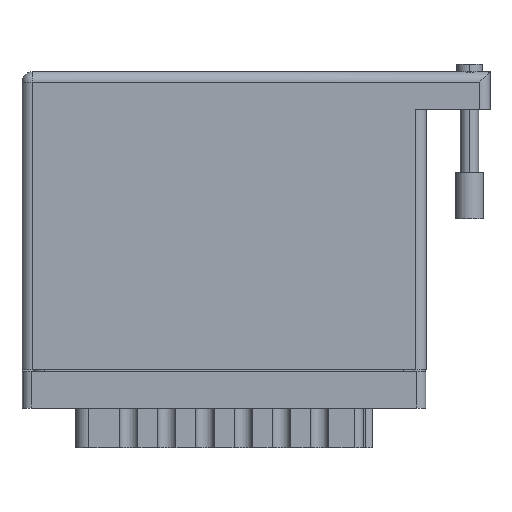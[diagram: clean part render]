
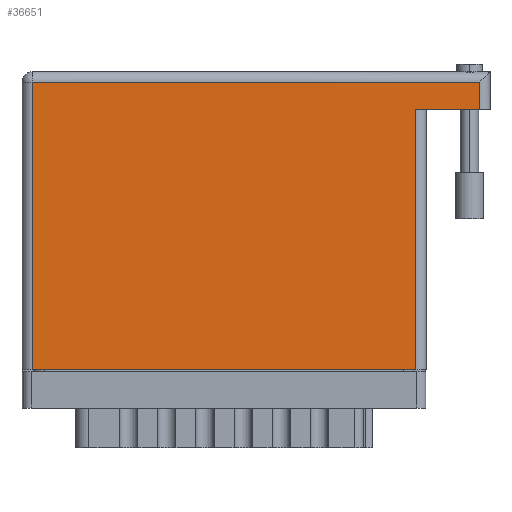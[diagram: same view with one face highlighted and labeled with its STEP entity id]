
A CAD part, front view. The second image highlights one B-rep face of the part: STEP entity #36651.
In plain terms, the highlighted face is planar.
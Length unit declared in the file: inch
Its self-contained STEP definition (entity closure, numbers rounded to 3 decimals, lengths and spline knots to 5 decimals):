
#3708 = ORIENTED_EDGE ( 'NONE', *, *, #39701, .T. ) ;
#4534 = EDGE_CURVE ( 'NONE', #19356, #83538, #9143, .T. ) ;
#5139 = ORIENTED_EDGE ( 'NONE', *, *, #76284, .T. ) ;
#6839 = DIRECTION ( 'NONE',  ( -1., 0., 0. ) ) ;
#7424 = DIRECTION ( 'NONE',  ( 0., 1., 0. ) ) ;
#9143 = LINE ( 'NONE', #72900, #36243 ) ;
#11621 = DIRECTION ( 'NONE',  ( -1., 0., 0. ) ) ;
#12824 = CARTESIAN_POINT ( 'NONE',  ( 0.07, 0., 0. ) ) ;
#16376 = DIRECTION ( 'NONE',  ( 0., -1., 0. ) ) ;
#19356 = VERTEX_POINT ( 'NONE', #27586 ) ;
#19974 = VERTEX_POINT ( 'NONE', #71896 ) ;
#22896 = DIRECTION ( 'NONE',  ( 1., 0., 0. ) ) ;
#23341 = DIRECTION ( 'NONE',  ( 0., 1., 0. ) ) ;
#24242 = LINE ( 'NONE', #28365, #34019 ) ;
#24522 = LINE ( 'NONE', #45507, #78759 ) ;
#26586 = LINE ( 'NONE', #85681, #79651 ) ;
#27586 = CARTESIAN_POINT ( 'NONE',  ( 2.685, 0., 0. ) ) ;
#28365 = CARTESIAN_POINT ( 'NONE',  ( 3.12, 2.03, 0. ) ) ;
#29286 = CARTESIAN_POINT ( 'NONE',  ( 0., 0., 0. ) ) ;
#30065 = VERTEX_POINT ( 'NONE', #12824 ) ;
#33862 = DIRECTION ( 'NONE',  ( 0., 0., -1. ) ) ;
#34019 = VECTOR ( 'NONE', #7424, 39.37008 ) ;
#36243 = VECTOR ( 'NONE', #23341, 39.37008 ) ;
#36651 = ADVANCED_FACE ( 'NONE', ( #40714 ), #82860, .F. ) ;
#38040 = CARTESIAN_POINT ( 'NONE',  ( 0.07, 1.96, 0. ) ) ;
#39701 = EDGE_CURVE ( 'NONE', #43799, #65156, #72883, .T. ) ;
#40714 = FACE_OUTER_BOUND ( 'NONE', #68778, .T. ) ;
#43799 = VERTEX_POINT ( 'NONE', #87037 ) ;
#45507 = CARTESIAN_POINT ( 'NONE',  ( 3.19, 1.774, 0. ) ) ;
#49966 = AXIS2_PLACEMENT_3D ( 'NONE', #54646, #33862, #6839 ) ;
#50435 = ORIENTED_EDGE ( 'NONE', *, *, #77606, .T. ) ;
#51267 = VECTOR ( 'NONE', #61161, 39.37008 ) ;
#53259 = CARTESIAN_POINT ( 'NONE',  ( 0., 1.96, 0. ) ) ;
#54646 = CARTESIAN_POINT ( 'NONE',  ( 0., 2.03, 0. ) ) ;
#59424 = ORIENTED_EDGE ( 'NONE', *, *, #87894, .F. ) ;
#61161 = DIRECTION ( 'NONE',  ( -1., 0., 0. ) ) ;
#62906 = EDGE_CURVE ( 'NONE', #65156, #30065, #26586, .T. ) ;
#65156 = VERTEX_POINT ( 'NONE', #38040 ) ;
#68778 = EDGE_LOOP ( 'NONE', ( #5139, #71581, #59424, #50435, #3708, #85687 ) ) ;
#68781 = VECTOR ( 'NONE', #22896, 39.37008 ) ;
#71581 = ORIENTED_EDGE ( 'NONE', *, *, #4534, .T. ) ;
#71896 = CARTESIAN_POINT ( 'NONE',  ( 3.12, 1.774, 0. ) ) ;
#72883 = LINE ( 'NONE', #53259, #51267 ) ;
#72900 = CARTESIAN_POINT ( 'NONE',  ( 2.685, 1.774, 0. ) ) ;
#76284 = EDGE_CURVE ( 'NONE', #30065, #19356, #87265, .T. ) ;
#77606 = EDGE_CURVE ( 'NONE', #19974, #43799, #24242, .T. ) ;
#78651 = CARTESIAN_POINT ( 'NONE',  ( 2.685, 1.774, 0. ) ) ;
#78759 = VECTOR ( 'NONE', #11621, 39.37008 ) ;
#79651 = VECTOR ( 'NONE', #16376, 39.37008 ) ;
#82860 = PLANE ( 'NONE',  #49966 ) ;
#83538 = VERTEX_POINT ( 'NONE', #78651 ) ;
#85681 = CARTESIAN_POINT ( 'NONE',  ( 0.07, 0., 0. ) ) ;
#85687 = ORIENTED_EDGE ( 'NONE', *, *, #62906, .T. ) ;
#87037 = CARTESIAN_POINT ( 'NONE',  ( 3.12, 1.96, 0. ) ) ;
#87265 = LINE ( 'NONE', #29286, #68781 ) ;
#87894 = EDGE_CURVE ( 'NONE', #19974, #83538, #24522, .T. ) ;
